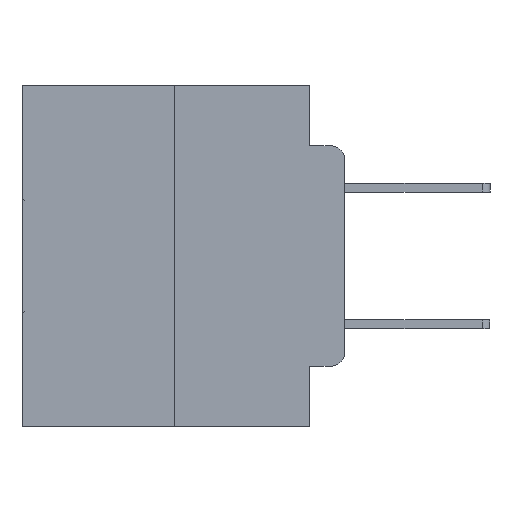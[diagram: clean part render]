
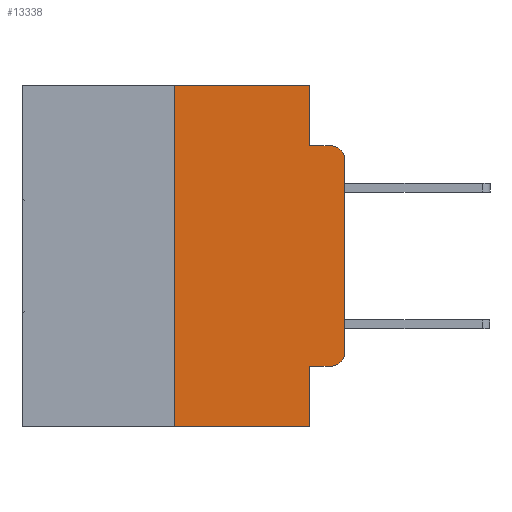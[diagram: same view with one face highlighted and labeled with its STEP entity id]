
A CAD part, left-side view. The second image highlights one B-rep face of the part: STEP entity #13338.
In plain terms, the highlighted planar face has unit normal (-1, 0, 0).
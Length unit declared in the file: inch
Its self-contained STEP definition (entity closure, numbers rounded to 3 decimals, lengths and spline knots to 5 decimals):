
#233 = LINE ( 'NONE', #4809, #11448 ) ;
#477 = VERTEX_POINT ( 'NONE', #3988 ) ;
#674 = LINE ( 'NONE', #27821, #24831 ) ;
#680 = EDGE_LOOP ( 'NONE', ( #27350, #1485, #8124, #2944, #29455, #3503, #18654, #12927, #11549, #21969 ) ) ;
#770 = DIRECTION ( 'NONE',  ( 0., -1., 0. ) ) ;
#1165 = VERTEX_POINT ( 'NONE', #9509 ) ;
#1425 = CARTESIAN_POINT ( 'NONE',  ( 0., 0.25, -0.5 ) ) ;
#1485 = ORIENTED_EDGE ( 'NONE', *, *, #3224, .T. ) ;
#1598 = EDGE_CURVE ( 'NONE', #1165, #6535, #29697, .T. ) ;
#1605 = EDGE_CURVE ( 'NONE', #1617, #16282, #233, .T. ) ;
#1617 = VERTEX_POINT ( 'NONE', #4733 ) ;
#1760 = CARTESIAN_POINT ( 'NONE',  ( 0., 0.02, -0.4115 ) ) ;
#2270 = DIRECTION ( 'NONE',  ( 0., 0., 1. ) ) ;
#2319 = VERTEX_POINT ( 'NONE', #5648 ) ;
#2786 = CARTESIAN_POINT ( 'NONE',  ( 0., 0.473, 0. ) ) ;
#2944 = ORIENTED_EDGE ( 'NONE', *, *, #25661, .F. ) ;
#3056 = VERTEX_POINT ( 'NONE', #8568 ) ;
#3224 = EDGE_CURVE ( 'NONE', #25538, #16282, #12866, .T. ) ;
#3503 = ORIENTED_EDGE ( 'NONE', *, *, #24122, .F. ) ;
#3908 = AXIS2_PLACEMENT_3D ( 'NONE', #8418, #24586, #10785 ) ;
#3988 = CARTESIAN_POINT ( 'NONE',  ( 0., 0., -0.3915 ) ) ;
#4219 = CARTESIAN_POINT ( 'NONE',  ( 0., 0.473, -0.5 ) ) ;
#4287 = VERTEX_POINT ( 'NONE', #1425 ) ;
#4324 = DIRECTION ( 'NONE',  ( 0., -1., 0. ) ) ;
#4688 = LINE ( 'NONE', #28660, #22596 ) ;
#4733 = CARTESIAN_POINT ( 'NONE',  ( 0., 0.051, -0.0885 ) ) ;
#4809 = CARTESIAN_POINT ( 'NONE',  ( 0., 0.051, -0.0885 ) ) ;
#4906 = DIRECTION ( 'NONE',  ( 0., -1., 0. ) ) ;
#5003 = DIRECTION ( 'NONE',  ( 0., -1., 0. ) ) ;
#5119 = VECTOR ( 'NONE', #5003, 39.37008 ) ;
#5426 = EDGE_CURVE ( 'NONE', #11635, #477, #25081, .T. ) ;
#5648 = CARTESIAN_POINT ( 'NONE',  ( 0., 0.051, -0.4115 ) ) ;
#6137 = CARTESIAN_POINT ( 'NONE',  ( 0., 0., 0. ) ) ;
#6535 = VERTEX_POINT ( 'NONE', #12564 ) ;
#6998 = DIRECTION ( 'NONE',  ( -1., 0., 0. ) ) ;
#7315 = DIRECTION ( 'NONE',  ( 0., 0., -1. ) ) ;
#7376 = VECTOR ( 'NONE', #7315, 39.37008 ) ;
#8029 = EDGE_CURVE ( 'NONE', #477, #25538, #11306, .T. ) ;
#8124 = ORIENTED_EDGE ( 'NONE', *, *, #1605, .F. ) ;
#8418 = CARTESIAN_POINT ( 'NONE',  ( 0., 0.473, 0. ) ) ;
#8515 = DIRECTION ( 'NONE',  ( 0., 0., 1. ) ) ;
#8568 = CARTESIAN_POINT ( 'NONE',  ( 0., 0.051, -0.5 ) ) ;
#8811 = DIRECTION ( 'NONE',  ( 0., 0., -1. ) ) ;
#9509 = CARTESIAN_POINT ( 'NONE',  ( 0., 0.25, 0. ) ) ;
#9694 = DIRECTION ( 'NONE',  ( 0., 0., -1. ) ) ;
#10203 = EDGE_CURVE ( 'NONE', #2319, #11635, #4688, .T. ) ;
#10546 = VECTOR ( 'NONE', #8515, 39.37008 ) ;
#10785 = DIRECTION ( 'NONE',  ( 0., 0., -1. ) ) ;
#11040 = AXIS2_PLACEMENT_3D ( 'NONE', #20926, #6998, #8811 ) ;
#11306 = LINE ( 'NONE', #6137, #10546 ) ;
#11428 = CARTESIAN_POINT ( 'NONE',  ( 0., 0.02, -0.0885 ) ) ;
#11448 = VECTOR ( 'NONE', #4906, 39.37008 ) ;
#11549 = ORIENTED_EDGE ( 'NONE', *, *, #10203, .T. ) ;
#11635 = VERTEX_POINT ( 'NONE', #1760 ) ;
#12325 = VECTOR ( 'NONE', #4324, 39.37008 ) ;
#12375 = DIRECTION ( 'NONE',  ( 0., 0., -1. ) ) ;
#12564 = CARTESIAN_POINT ( 'NONE',  ( 0., 0.051, 0. ) ) ;
#12866 = CIRCLE ( 'NONE', #11040, 0.02 ) ;
#12927 = ORIENTED_EDGE ( 'NONE', *, *, #14924, .F. ) ;
#13338 = ADVANCED_FACE ( 'NONE', ( #13456 ), #20058, .F. ) ;
#13456 = FACE_OUTER_BOUND ( 'NONE', #680, .T. ) ;
#13632 = CARTESIAN_POINT ( 'NONE',  ( 0., 0.02, -0.3915 ) ) ;
#13811 = CARTESIAN_POINT ( 'NONE',  ( 0., 0., -0.1085 ) ) ;
#14628 = CARTESIAN_POINT ( 'NONE',  ( 0., 0.051, 0. ) ) ;
#14924 = EDGE_CURVE ( 'NONE', #2319, #3056, #26581, .T. ) ;
#16282 = VERTEX_POINT ( 'NONE', #11428 ) ;
#16363 = AXIS2_PLACEMENT_3D ( 'NONE', #13632, #18030, #9694 ) ;
#18030 = DIRECTION ( 'NONE',  ( -1., 0., 0. ) ) ;
#18477 = LINE ( 'NONE', #4219, #12325 ) ;
#18654 = ORIENTED_EDGE ( 'NONE', *, *, #21897, .T. ) ;
#20058 = PLANE ( 'NONE',  #3908 ) ;
#20926 = CARTESIAN_POINT ( 'NONE',  ( 0., 0.02, -0.1085 ) ) ;
#21250 = CARTESIAN_POINT ( 'NONE',  ( 0., 0.051, 0. ) ) ;
#21897 = EDGE_CURVE ( 'NONE', #4287, #3056, #18477, .T. ) ;
#21969 = ORIENTED_EDGE ( 'NONE', *, *, #5426, .T. ) ;
#22596 = VECTOR ( 'NONE', #770, 39.37008 ) ;
#24122 = EDGE_CURVE ( 'NONE', #4287, #1165, #674, .T. ) ;
#24586 = DIRECTION ( 'NONE',  ( 1., 0., 0. ) ) ;
#24831 = VECTOR ( 'NONE', #2270, 39.37008 ) ;
#25081 = CIRCLE ( 'NONE', #16363, 0.02 ) ;
#25096 = LINE ( 'NONE', #21250, #7376 ) ;
#25538 = VERTEX_POINT ( 'NONE', #13811 ) ;
#25661 = EDGE_CURVE ( 'NONE', #6535, #1617, #25096, .T. ) ;
#25889 = VECTOR ( 'NONE', #12375, 39.37008 ) ;
#26581 = LINE ( 'NONE', #14628, #25889 ) ;
#27350 = ORIENTED_EDGE ( 'NONE', *, *, #8029, .T. ) ;
#27821 = CARTESIAN_POINT ( 'NONE',  ( 0., 0.25, 0. ) ) ;
#28660 = CARTESIAN_POINT ( 'NONE',  ( 0., 0.051, -0.4115 ) ) ;
#29455 = ORIENTED_EDGE ( 'NONE', *, *, #1598, .F. ) ;
#29697 = LINE ( 'NONE', #2786, #5119 ) ;
